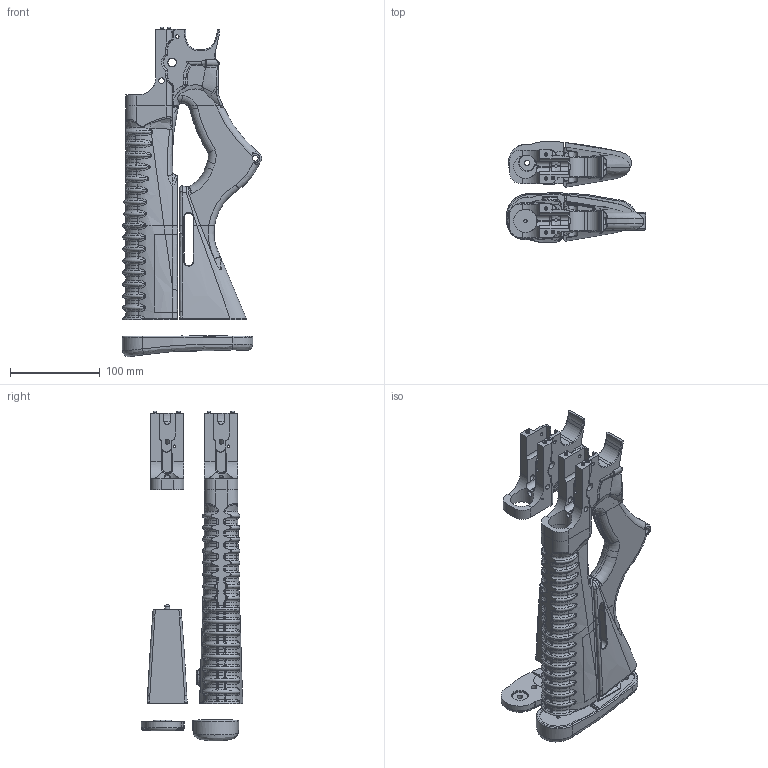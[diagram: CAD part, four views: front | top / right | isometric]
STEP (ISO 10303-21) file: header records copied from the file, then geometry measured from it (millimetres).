
FILE_DESCRIPTION(/* description */ (''),/* implementation_level */ '2;1');
FILE_NAME(/* name */ 'AA2 (v10~recovered).step',/* time_stamp */ '2020-05-20T22:27:03-05:00',/* author */ (''),/* organization */ (''),/* preprocessor_version */ 'ST-DEVELOPER v18.1',/* originating_system */ 'Autodesk Translation Framework v9.3.0.1241',/* authorisation */ '');
FILE_SCHEMA (('AUTOMOTIVE_DESIGN { 1 0 10303 214 3 1 1 }'));
Products named in the file (1): AA2 (v10~recovered)
Bounding box: 154.65 x 112.77 x 366.25 mm (x, y, z)
Volume: 1067242.3 mm3; surface area: 254238.6 mm2
Topology: 11 solids, 21 shells, 2646 faces, 7182 edges, 4683 vertices
Faces by surface type: plane 1009, bspline 866, cylinder 554, torus 197, sphere 15, cone 5
Full cylindrical faces by diameter (mm): 0.508 x2, 2.103 x1, 2.54 x1, 3.175 x6, 3.2 x2, 3.969 x4, 4 x8, 4.826 x5, 4.9 x1, 5 x6, 5.004 x26, 5.334 x6, 6.1 x5, 6.35 x8, 6.477 x1, 6.807 x2, 6.858 x1, 7 x1, 7.036 x2, 7.493 x2, 8.509 x1, 8.733 x1, 9.525 x4, 10 x2, 13 x1, 18.721 x1, 25.95 x4
Entity records: 169887 total; most frequent: CARTESIAN_POINT 109842, ORIENTED_EDGE 14344, DIRECTION 9467, EDGE_CURVE 7172, VERTEX_POINT 4687, AXIS2_PLACEMENT_3D 3277, LINE 2913, VECTOR 2913
